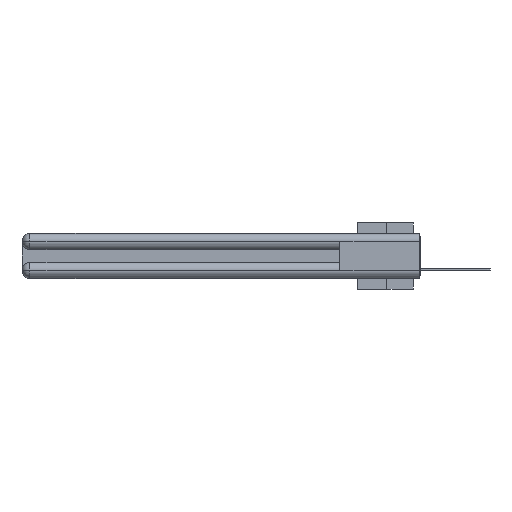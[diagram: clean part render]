
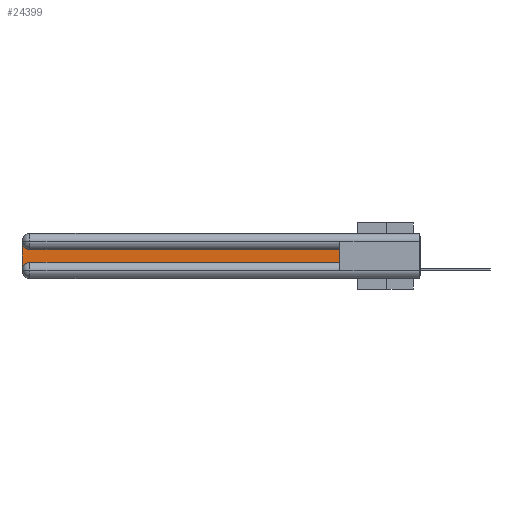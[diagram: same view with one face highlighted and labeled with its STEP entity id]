
A CAD part, left-side view. The second image highlights one B-rep face of the part: STEP entity #24399.
In plain terms, the highlighted planar face has unit normal (-1, 0, 0).
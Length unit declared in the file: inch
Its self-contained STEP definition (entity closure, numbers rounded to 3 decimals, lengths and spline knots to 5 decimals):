
#1469 = CARTESIAN_POINT ( 'NONE',  ( 0.075, 0.6, -0.1225 ) ) ;
#1917 = CARTESIAN_POINT ( 'NONE',  ( 0.075, 3., -0.0625 ) ) ;
#1975 = VERTEX_POINT ( 'NONE', #1917 ) ;
#1982 = VERTEX_POINT ( 'NONE', #31045 ) ;
#2064 = DIRECTION ( 'NONE',  ( 0., 0., 1. ) ) ;
#2158 = EDGE_CURVE ( 'NONE', #25902, #31679, #19372, .T. ) ;
#2730 = DIRECTION ( 'NONE',  ( 1., 0., 0. ) ) ;
#2935 = AXIS2_PLACEMENT_3D ( 'NONE', #19953, #2974, #29666 ) ;
#2974 = DIRECTION ( 'NONE',  ( 1., 0., 0. ) ) ;
#4804 = LINE ( 'NONE', #9201, #28299 ) ;
#4985 = CIRCLE ( 'NONE', #2935, 0.06 ) ;
#5092 = LINE ( 'NONE', #29853, #14301 ) ;
#5355 = EDGE_CURVE ( 'NONE', #12406, #1982, #4985, .T. ) ;
#6599 = CARTESIAN_POINT ( 'NONE',  ( 0.075, 2.94, -0.1225 ) ) ;
#6936 = AXIS2_PLACEMENT_3D ( 'NONE', #9847, #2730, #21397 ) ;
#6997 = CIRCLE ( 'NONE', #31818, 0.06 ) ;
#7235 = CARTESIAN_POINT ( 'NONE',  ( 0.075, 0.6, -0.1225 ) ) ;
#7371 = VECTOR ( 'NONE', #30930, 39.37008 ) ;
#7484 = VERTEX_POINT ( 'NONE', #6599 ) ;
#7960 = ORIENTED_EDGE ( 'NONE', *, *, #20744, .T. ) ;
#9201 = CARTESIAN_POINT ( 'NONE',  ( 0.075, 3., -0.2175 ) ) ;
#9847 = CARTESIAN_POINT ( 'NONE',  ( 0.075, 3., -0.1225 ) ) ;
#9973 = EDGE_CURVE ( 'NONE', #31679, #7484, #23641, .T. ) ;
#12406 = VERTEX_POINT ( 'NONE', #15642 ) ;
#13478 = ORIENTED_EDGE ( 'NONE', *, *, #9973, .T. ) ;
#14095 = VECTOR ( 'NONE', #2064, 39.37008 ) ;
#14254 = EDGE_LOOP ( 'NONE', ( #13478, #7960, #20084, #17312, #18493, #28506 ) ) ;
#14301 = VECTOR ( 'NONE', #30339, 39.37008 ) ;
#14728 = FACE_OUTER_BOUND ( 'NONE', #14254, .T. ) ;
#15236 = EDGE_CURVE ( 'NONE', #1975, #12406, #4804, .T. ) ;
#15642 = CARTESIAN_POINT ( 'NONE',  ( 0.075, 3., -0.2775 ) ) ;
#17312 = ORIENTED_EDGE ( 'NONE', *, *, #5355, .T. ) ;
#18493 = ORIENTED_EDGE ( 'NONE', *, *, #29391, .T. ) ;
#18784 = DIRECTION ( 'NONE',  ( 1., 0., 0. ) ) ;
#19372 = LINE ( 'NONE', #27132, #14095 ) ;
#19953 = CARTESIAN_POINT ( 'NONE',  ( 0.075, 2.94, -0.2775 ) ) ;
#20084 = ORIENTED_EDGE ( 'NONE', *, *, #15236, .T. ) ;
#20744 = EDGE_CURVE ( 'NONE', #7484, #1975, #6997, .T. ) ;
#21397 = DIRECTION ( 'NONE',  ( 0., 0., -1. ) ) ;
#23641 = LINE ( 'NONE', #1469, #7371 ) ;
#23654 = CARTESIAN_POINT ( 'NONE',  ( 0.075, 2.94, -0.0625 ) ) ;
#23917 = DIRECTION ( 'NONE',  ( 0., 0., -1. ) ) ;
#24399 = ADVANCED_FACE ( 'NONE', ( #14728 ), #26409, .F. ) ;
#25897 = CARTESIAN_POINT ( 'NONE',  ( 0.075, 0.6, -0.2175 ) ) ;
#25902 = VERTEX_POINT ( 'NONE', #25897 ) ;
#26379 = DIRECTION ( 'NONE',  ( 0., 0., -1. ) ) ;
#26409 = PLANE ( 'NONE',  #6936 ) ;
#27132 = CARTESIAN_POINT ( 'NONE',  ( 0.075, 0.6, -0.2175 ) ) ;
#28299 = VECTOR ( 'NONE', #23917, 39.37008 ) ;
#28506 = ORIENTED_EDGE ( 'NONE', *, *, #2158, .T. ) ;
#29391 = EDGE_CURVE ( 'NONE', #1982, #25902, #5092, .T. ) ;
#29666 = DIRECTION ( 'NONE',  ( 0., 0., -1. ) ) ;
#29853 = CARTESIAN_POINT ( 'NONE',  ( 0.075, 0.6, -0.2175 ) ) ;
#30339 = DIRECTION ( 'NONE',  ( 0., -1., 0. ) ) ;
#30930 = DIRECTION ( 'NONE',  ( 0., 1., 0. ) ) ;
#31045 = CARTESIAN_POINT ( 'NONE',  ( 0.075, 2.94, -0.2175 ) ) ;
#31679 = VERTEX_POINT ( 'NONE', #7235 ) ;
#31818 = AXIS2_PLACEMENT_3D ( 'NONE', #23654, #18784, #26379 ) ;
